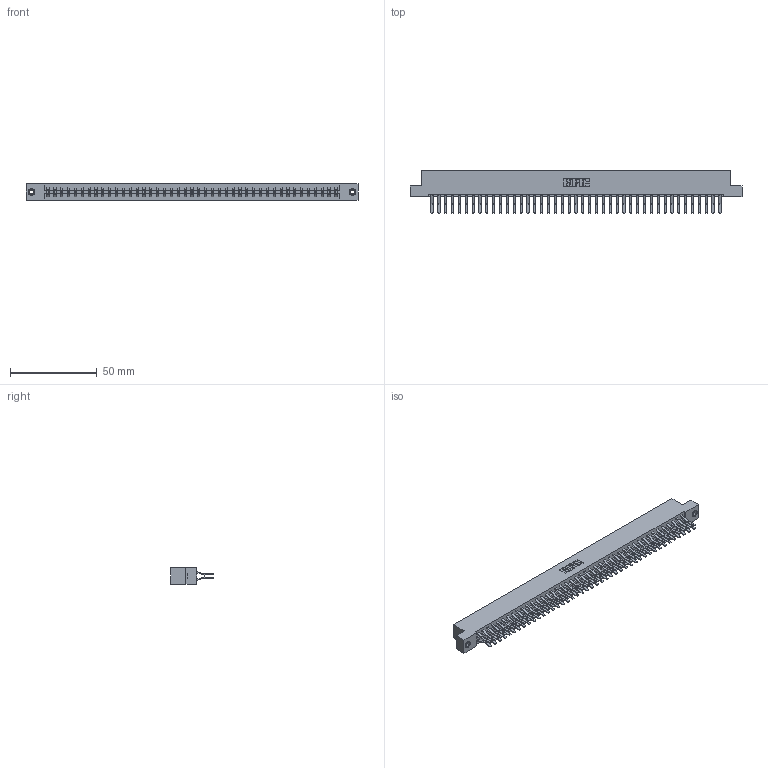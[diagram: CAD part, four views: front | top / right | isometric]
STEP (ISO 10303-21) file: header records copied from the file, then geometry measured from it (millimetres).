
FILE_DESCRIPTION (( 'STEP AP203' ), '1' );
FILE_NAME ('333-086-560-208.STEP', '2018-08-05T07:07:55', ( '' ), ( '' ), 'SwSTEP 2.0', 'SolidWorks 2016', '' );
FILE_SCHEMA (( 'CONFIG_CONTROL_DESIGN' ));
Length unit declared in the file: inch
Products named in the file (4): 333 Part_Flush - .156 Dia - TI; 345-292-001_560 Tail; 345-250-001_345-250-003-102; 333-086-560-208
Assembly tree (89 placements, depth 2):
  333-086-560-208
    333 Part_Flush - .156 Dia - TI
    345-292-001_560 Tail  x86
    345-250-001_345-250-003-102  x2
Bounding box: 191.92 x 24.78 x 9.4 mm (x, y, z)
Volume: 20160.7 mm3; surface area: 25475.5 mm2
Topology: 89 solids, 89 shells, 4818 faces, 14293 edges, 9406 vertices
Faces by surface type: plane 3198, cylinder 1604, cone 12, torus 4
Entity records: 28808 total; most frequent: CARTESIAN_POINT 4757, ORIENTED_EDGE 4686, DIRECTION 4097, EDGE_CURVE 2343, LINE 2191, VECTOR 2191, VERTEX_POINT 1556, AXIS2_PLACEMENT_3D 953
